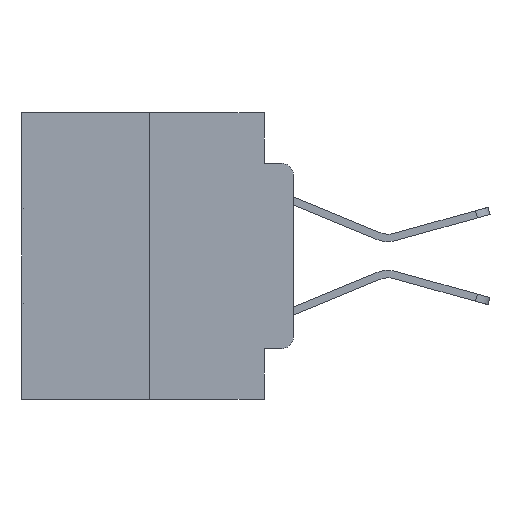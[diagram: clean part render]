
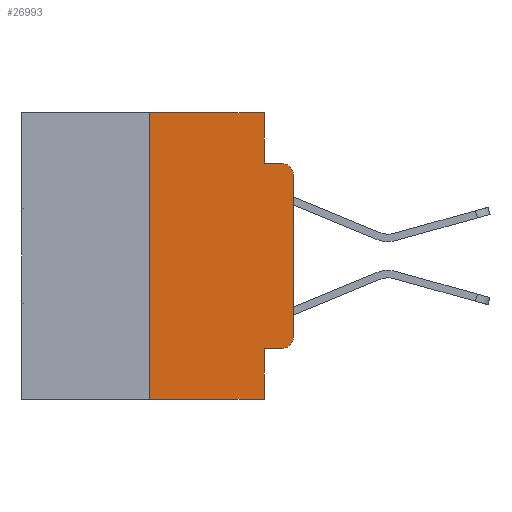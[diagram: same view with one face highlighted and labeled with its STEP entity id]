
A CAD part, left-side view. The second image highlights one B-rep face of the part: STEP entity #26993.
In plain terms, the highlighted planar face has unit normal (-1, 0, 0).
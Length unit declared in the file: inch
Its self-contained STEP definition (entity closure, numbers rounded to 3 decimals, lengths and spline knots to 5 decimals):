
#349 = LINE ( 'NONE', #13129, #11730 ) ;
#463 = DIRECTION ( 'NONE',  ( 1., 0., 0. ) ) ;
#1279 = VERTEX_POINT ( 'NONE', #27660 ) ;
#1450 = AXIS2_PLACEMENT_3D ( 'NONE', #13329, #28830, #15593 ) ;
#1838 = VECTOR ( 'NONE', #2169, 39.37008 ) ;
#1885 = EDGE_CURVE ( 'NONE', #14656, #5265, #5013, .T. ) ;
#2034 = VECTOR ( 'NONE', #24190, 39.37008 ) ;
#2169 = DIRECTION ( 'NONE',  ( 0., 0., -1. ) ) ;
#2539 = FACE_OUTER_BOUND ( 'NONE', #22401, .T. ) ;
#3073 = VERTEX_POINT ( 'NONE', #4781 ) ;
#3435 = EDGE_CURVE ( 'NONE', #18953, #14656, #6701, .T. ) ;
#4781 = CARTESIAN_POINT ( 'NONE',  ( 0., 0.051, -0.5 ) ) ;
#5013 = CIRCLE ( 'NONE', #7682, 0.02 ) ;
#5181 = CARTESIAN_POINT ( 'NONE',  ( 0., 0.25, 0. ) ) ;
#5265 = VERTEX_POINT ( 'NONE', #20799 ) ;
#5313 = DIRECTION ( 'NONE',  ( -1., 0., 0. ) ) ;
#5679 = LINE ( 'NONE', #15957, #22851 ) ;
#5781 = ORIENTED_EDGE ( 'NONE', *, *, #25051, .F. ) ;
#5995 = VECTOR ( 'NONE', #25901, 39.37008 ) ;
#6247 = VERTEX_POINT ( 'NONE', #14857 ) ;
#6326 = CARTESIAN_POINT ( 'NONE',  ( 0., 0.051, 0. ) ) ;
#6701 = LINE ( 'NONE', #8063, #5995 ) ;
#6740 = EDGE_CURVE ( 'NONE', #21058, #6247, #11050, .T. ) ;
#7032 = CARTESIAN_POINT ( 'NONE',  ( 0., 0., -0.1085 ) ) ;
#7094 = EDGE_CURVE ( 'NONE', #1279, #18953, #21204, .T. ) ;
#7199 = ORIENTED_EDGE ( 'NONE', *, *, #13103, .F. ) ;
#7682 = AXIS2_PLACEMENT_3D ( 'NONE', #18775, #5313, #20994 ) ;
#8063 = CARTESIAN_POINT ( 'NONE',  ( 0., 0., 0. ) ) ;
#9198 = CARTESIAN_POINT ( 'NONE',  ( 0., 0.051, -0.0885 ) ) ;
#9376 = LINE ( 'NONE', #23180, #26425 ) ;
#10711 = LINE ( 'NONE', #12466, #21224 ) ;
#11050 = LINE ( 'NONE', #23312, #17042 ) ;
#11593 = EDGE_CURVE ( 'NONE', #26872, #1279, #349, .T. ) ;
#11730 = VECTOR ( 'NONE', #15396, 39.37008 ) ;
#11749 = ORIENTED_EDGE ( 'NONE', *, *, #16125, .F. ) ;
#11769 = VERTEX_POINT ( 'NONE', #9198 ) ;
#12466 = CARTESIAN_POINT ( 'NONE',  ( 0., 0.473, -0.5 ) ) ;
#13103 = EDGE_CURVE ( 'NONE', #26872, #3073, #19347, .T. ) ;
#13129 = CARTESIAN_POINT ( 'NONE',  ( 0., 0.051, -0.4115 ) ) ;
#13329 = CARTESIAN_POINT ( 'NONE',  ( 0., 0.02, -0.3915 ) ) ;
#13494 = ORIENTED_EDGE ( 'NONE', *, *, #3435, .T. ) ;
#14175 = ORIENTED_EDGE ( 'NONE', *, *, #6740, .F. ) ;
#14203 = ORIENTED_EDGE ( 'NONE', *, *, #1885, .T. ) ;
#14582 = ORIENTED_EDGE ( 'NONE', *, *, #7094, .T. ) ;
#14656 = VERTEX_POINT ( 'NONE', #7032 ) ;
#14733 = DIRECTION ( 'NONE',  ( 0., -1., 0. ) ) ;
#14857 = CARTESIAN_POINT ( 'NONE',  ( 0., 0.051, 0. ) ) ;
#15396 = DIRECTION ( 'NONE',  ( 0., -1., 0. ) ) ;
#15593 = DIRECTION ( 'NONE',  ( 0., 0., -1. ) ) ;
#15957 = CARTESIAN_POINT ( 'NONE',  ( 0., 0.051, -0.0885 ) ) ;
#16125 = EDGE_CURVE ( 'NONE', #21162, #21058, #9376, .T. ) ;
#16326 = DIRECTION ( 'NONE',  ( 0., 0., -1. ) ) ;
#17042 = VECTOR ( 'NONE', #25514, 39.37008 ) ;
#18202 = DIRECTION ( 'NONE',  ( 0., -1., 0. ) ) ;
#18424 = ORIENTED_EDGE ( 'NONE', *, *, #22471, .T. ) ;
#18743 = ORIENTED_EDGE ( 'NONE', *, *, #22086, .F. ) ;
#18775 = CARTESIAN_POINT ( 'NONE',  ( 0., 0.02, -0.1085 ) ) ;
#18953 = VERTEX_POINT ( 'NONE', #23584 ) ;
#18989 = AXIS2_PLACEMENT_3D ( 'NONE', #20697, #463, #16326 ) ;
#19347 = LINE ( 'NONE', #6326, #2034 ) ;
#19854 = LINE ( 'NONE', #28969, #1838 ) ;
#20697 = CARTESIAN_POINT ( 'NONE',  ( 0., 0.473, 0. ) ) ;
#20799 = CARTESIAN_POINT ( 'NONE',  ( 0., 0.02, -0.0885 ) ) ;
#20994 = DIRECTION ( 'NONE',  ( 0., 0., -1. ) ) ;
#21058 = VERTEX_POINT ( 'NONE', #5181 ) ;
#21162 = VERTEX_POINT ( 'NONE', #27971 ) ;
#21204 = CIRCLE ( 'NONE', #1450, 0.02 ) ;
#21224 = VECTOR ( 'NONE', #14733, 39.37008 ) ;
#22086 = EDGE_CURVE ( 'NONE', #6247, #11769, #19854, .T. ) ;
#22401 = EDGE_LOOP ( 'NONE', ( #13494, #14203, #5781, #18743, #14175, #11749, #18424, #7199, #25679, #14582 ) ) ;
#22471 = EDGE_CURVE ( 'NONE', #21162, #3073, #10711, .T. ) ;
#22851 = VECTOR ( 'NONE', #18202, 39.37008 ) ;
#23180 = CARTESIAN_POINT ( 'NONE',  ( 0., 0.25, 0. ) ) ;
#23312 = CARTESIAN_POINT ( 'NONE',  ( 0., 0.473, 0. ) ) ;
#23584 = CARTESIAN_POINT ( 'NONE',  ( 0., 0., -0.3915 ) ) ;
#24190 = DIRECTION ( 'NONE',  ( 0., 0., -1. ) ) ;
#24669 = CARTESIAN_POINT ( 'NONE',  ( 0., 0.051, -0.4115 ) ) ;
#25051 = EDGE_CURVE ( 'NONE', #11769, #5265, #5679, .T. ) ;
#25396 = DIRECTION ( 'NONE',  ( 0., 0., 1. ) ) ;
#25514 = DIRECTION ( 'NONE',  ( 0., -1., 0. ) ) ;
#25679 = ORIENTED_EDGE ( 'NONE', *, *, #11593, .T. ) ;
#25901 = DIRECTION ( 'NONE',  ( 0., 0., 1. ) ) ;
#26425 = VECTOR ( 'NONE', #25396, 39.37008 ) ;
#26872 = VERTEX_POINT ( 'NONE', #24669 ) ;
#26993 = ADVANCED_FACE ( 'NONE', ( #2539 ), #27342, .F. ) ;
#27342 = PLANE ( 'NONE',  #18989 ) ;
#27660 = CARTESIAN_POINT ( 'NONE',  ( 0., 0.02, -0.4115 ) ) ;
#27971 = CARTESIAN_POINT ( 'NONE',  ( 0., 0.25, -0.5 ) ) ;
#28830 = DIRECTION ( 'NONE',  ( -1., 0., 0. ) ) ;
#28969 = CARTESIAN_POINT ( 'NONE',  ( 0., 0.051, 0. ) ) ;
